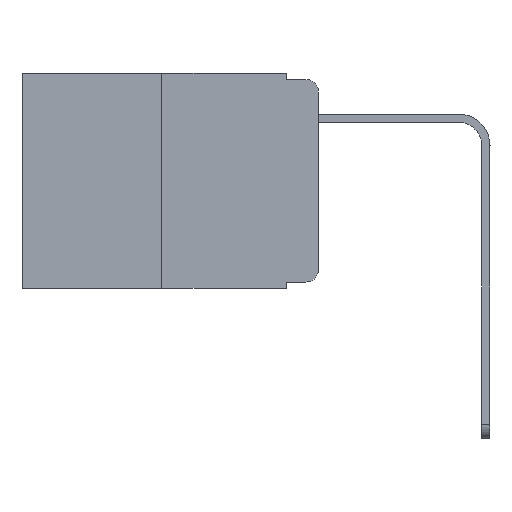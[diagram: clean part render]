
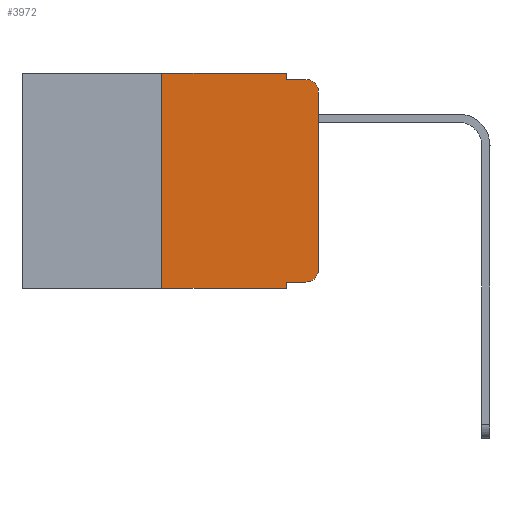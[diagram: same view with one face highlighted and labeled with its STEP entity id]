
A CAD part, left-side view. The second image highlights one B-rep face of the part: STEP entity #3972.
In plain terms, the highlighted planar face has unit normal (-1, 0, 0).
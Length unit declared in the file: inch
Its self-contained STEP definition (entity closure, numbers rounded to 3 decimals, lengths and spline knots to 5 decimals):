
#46 = CARTESIAN_POINT ( 'NONE',  ( 0., 0.473, -0.343 ) ) ;
#166 = CARTESIAN_POINT ( 'NONE',  ( 0., 0., -0.03 ) ) ;
#209 = DIRECTION ( 'NONE',  ( 0., -1., 0. ) ) ;
#349 = CARTESIAN_POINT ( 'NONE',  ( 0., 0.02, -0.313 ) ) ;
#578 = CARTESIAN_POINT ( 'NONE',  ( 0., 0.051, 0. ) ) ;
#742 = LINE ( 'NONE', #2053, #4917 ) ;
#907 = CARTESIAN_POINT ( 'NONE',  ( 0., 0.051, -0.01 ) ) ;
#1067 = DIRECTION ( 'NONE',  ( 0., 0., 1. ) ) ;
#1107 = ORIENTED_EDGE ( 'NONE', *, *, #1417, .T. ) ;
#1194 = DIRECTION ( 'NONE',  ( -1., 0., 0. ) ) ;
#1417 = EDGE_CURVE ( 'NONE', #6544, #5286, #8983, .T. ) ;
#1762 = ORIENTED_EDGE ( 'NONE', *, *, #2651, .F. ) ;
#1951 = ORIENTED_EDGE ( 'NONE', *, *, #7908, .T. ) ;
#2053 = CARTESIAN_POINT ( 'NONE',  ( 0., 0.051, -0.333 ) ) ;
#2078 = CARTESIAN_POINT ( 'NONE',  ( 0., 0.25, -0.343 ) ) ;
#2267 = ORIENTED_EDGE ( 'NONE', *, *, #8637, .F. ) ;
#2651 = EDGE_CURVE ( 'NONE', #6346, #6735, #10664, .T. ) ;
#2742 = VERTEX_POINT ( 'NONE', #5702 ) ;
#2747 = EDGE_CURVE ( 'NONE', #2742, #10273, #5681, .T. ) ;
#2764 = DIRECTION ( 'NONE',  ( 0., -1., 0. ) ) ;
#2816 = CIRCLE ( 'NONE', #5508, 0.02 ) ;
#3136 = VECTOR ( 'NONE', #2764, 39.37008 ) ;
#3571 = ORIENTED_EDGE ( 'NONE', *, *, #9663, .T. ) ;
#3644 = DIRECTION ( 'NONE',  ( 0., 0., -1. ) ) ;
#3651 = CARTESIAN_POINT ( 'NONE',  ( 0., 0.02, -0.03 ) ) ;
#3667 = LINE ( 'NONE', #907, #3136 ) ;
#3972 = ADVANCED_FACE ( 'NONE', ( #4369 ), #8995, .F. ) ;
#4043 = DIRECTION ( 'NONE',  ( 0., 0., -1. ) ) ;
#4189 = ORIENTED_EDGE ( 'NONE', *, *, #4972, .F. ) ;
#4268 = CARTESIAN_POINT ( 'NONE',  ( 0., 0.02, -0.333 ) ) ;
#4297 = AXIS2_PLACEMENT_3D ( 'NONE', #349, #5406, #3644 ) ;
#4369 = FACE_OUTER_BOUND ( 'NONE', #6115, .T. ) ;
#4615 = EDGE_CURVE ( 'NONE', #2742, #6544, #742, .T. ) ;
#4635 = CARTESIAN_POINT ( 'NONE',  ( 0., 0.25, 0. ) ) ;
#4779 = VERTEX_POINT ( 'NONE', #4852 ) ;
#4836 = VECTOR ( 'NONE', #8646, 39.37008 ) ;
#4852 = CARTESIAN_POINT ( 'NONE',  ( 0., 0.02, -0.01 ) ) ;
#4917 = VECTOR ( 'NONE', #209, 39.37008 ) ;
#4972 = EDGE_CURVE ( 'NONE', #5695, #4779, #3667, .T. ) ;
#5182 = DIRECTION ( 'NONE',  ( 0., -1., 0. ) ) ;
#5281 = CARTESIAN_POINT ( 'NONE',  ( 0., 0.051, -0.01 ) ) ;
#5286 = VERTEX_POINT ( 'NONE', #8122 ) ;
#5406 = DIRECTION ( 'NONE',  ( -1., 0., 0. ) ) ;
#5508 = AXIS2_PLACEMENT_3D ( 'NONE', #3651, #1194, #7930 ) ;
#5681 = LINE ( 'NONE', #578, #7726 ) ;
#5695 = VERTEX_POINT ( 'NONE', #5281 ) ;
#5702 = CARTESIAN_POINT ( 'NONE',  ( 0., 0.051, -0.333 ) ) ;
#5737 = CARTESIAN_POINT ( 'NONE',  ( 0., 0.051, 0. ) ) ;
#5906 = ORIENTED_EDGE ( 'NONE', *, *, #9327, .T. ) ;
#6115 = EDGE_LOOP ( 'NONE', ( #5906, #1951, #4189, #2267, #1762, #7199, #3571, #9300, #6687, #1107 ) ) ;
#6346 = VERTEX_POINT ( 'NONE', #8829 ) ;
#6476 = DIRECTION ( 'NONE',  ( 1., 0., 0. ) ) ;
#6544 = VERTEX_POINT ( 'NONE', #4268 ) ;
#6687 = ORIENTED_EDGE ( 'NONE', *, *, #4615, .T. ) ;
#6735 = VERTEX_POINT ( 'NONE', #5737 ) ;
#6902 = VERTEX_POINT ( 'NONE', #2078 ) ;
#6996 = VECTOR ( 'NONE', #9500, 39.37008 ) ;
#7199 = ORIENTED_EDGE ( 'NONE', *, *, #10606, .F. ) ;
#7425 = LINE ( 'NONE', #10598, #4836 ) ;
#7726 = VECTOR ( 'NONE', #10850, 39.37008 ) ;
#7908 = EDGE_CURVE ( 'NONE', #8761, #4779, #2816, .T. ) ;
#7930 = DIRECTION ( 'NONE',  ( 0., 0., -1. ) ) ;
#8122 = CARTESIAN_POINT ( 'NONE',  ( 0., 0., -0.313 ) ) ;
#8409 = VECTOR ( 'NONE', #5182, 39.37008 ) ;
#8467 = CARTESIAN_POINT ( 'NONE',  ( 0., 0.051, -0.343 ) ) ;
#8501 = VECTOR ( 'NONE', #9061, 39.37008 ) ;
#8505 = LINE ( 'NONE', #9739, #9580 ) ;
#8637 = EDGE_CURVE ( 'NONE', #6735, #5695, #7425, .T. ) ;
#8646 = DIRECTION ( 'NONE',  ( 0., 0., -1. ) ) ;
#8696 = CARTESIAN_POINT ( 'NONE',  ( 0., 0.473, 0. ) ) ;
#8761 = VERTEX_POINT ( 'NONE', #166 ) ;
#8829 = CARTESIAN_POINT ( 'NONE',  ( 0., 0.25, 0. ) ) ;
#8983 = CIRCLE ( 'NONE', #4297, 0.02 ) ;
#8995 = PLANE ( 'NONE',  #10970 ) ;
#9061 = DIRECTION ( 'NONE',  ( 0., 0., 1. ) ) ;
#9300 = ORIENTED_EDGE ( 'NONE', *, *, #2747, .F. ) ;
#9327 = EDGE_CURVE ( 'NONE', #5286, #8761, #8505, .T. ) ;
#9500 = DIRECTION ( 'NONE',  ( 0., -1., 0. ) ) ;
#9578 = LINE ( 'NONE', #4635, #8501 ) ;
#9580 = VECTOR ( 'NONE', #1067, 39.37008 ) ;
#9663 = EDGE_CURVE ( 'NONE', #6902, #10273, #10617, .T. ) ;
#9739 = CARTESIAN_POINT ( 'NONE',  ( 0., 0., 0. ) ) ;
#9906 = CARTESIAN_POINT ( 'NONE',  ( 0., 0.473, 0. ) ) ;
#10273 = VERTEX_POINT ( 'NONE', #8467 ) ;
#10598 = CARTESIAN_POINT ( 'NONE',  ( 0., 0.051, 0. ) ) ;
#10606 = EDGE_CURVE ( 'NONE', #6902, #6346, #9578, .T. ) ;
#10617 = LINE ( 'NONE', #46, #6996 ) ;
#10664 = LINE ( 'NONE', #8696, #8409 ) ;
#10850 = DIRECTION ( 'NONE',  ( 0., 0., -1. ) ) ;
#10970 = AXIS2_PLACEMENT_3D ( 'NONE', #9906, #6476, #4043 ) ;
